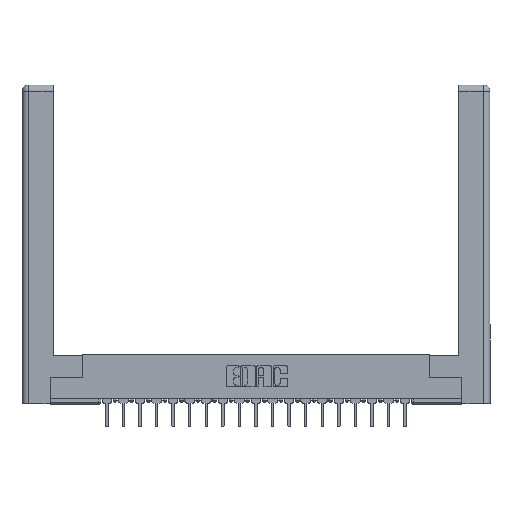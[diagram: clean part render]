
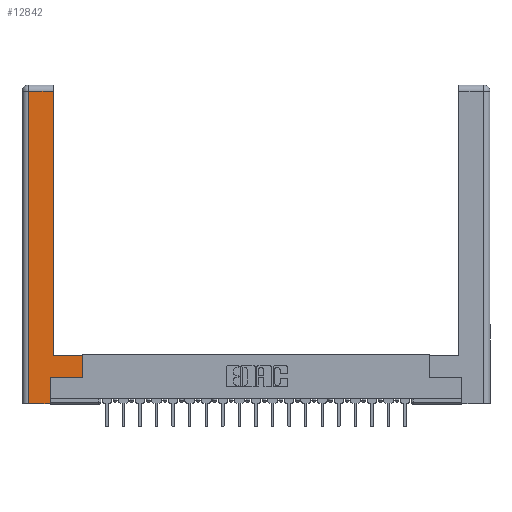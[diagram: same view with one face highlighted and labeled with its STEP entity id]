
A CAD part, top view. The second image highlights one B-rep face of the part: STEP entity #12842.
In plain terms, the highlighted planar face has unit normal (0, 0, 1).
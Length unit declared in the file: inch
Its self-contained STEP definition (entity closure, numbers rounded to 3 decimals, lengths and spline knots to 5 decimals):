
#192 = DIRECTION ( 'NONE',  ( 0., 1., 0. ) ) ;
#274 = CARTESIAN_POINT ( 'NONE',  ( 0.0615, 2.94, 0. ) ) ;
#944 = EDGE_CURVE ( 'NONE', #20094, #19150, #2194, .T. ) ;
#992 = ORIENTED_EDGE ( 'NONE', *, *, #944, .T. ) ;
#1923 = LINE ( 'NONE', #274, #16390 ) ;
#2165 = VERTEX_POINT ( 'NONE', #3200 ) ;
#2194 = LINE ( 'NONE', #18805, #19757 ) ;
#3169 = DIRECTION ( 'NONE',  ( 0., 1., 0. ) ) ;
#3200 = CARTESIAN_POINT ( 'NONE',  ( 0.295, 0.45, 0. ) ) ;
#3791 = VERTEX_POINT ( 'NONE', #3853 ) ;
#3798 = VECTOR ( 'NONE', #8963, 39.37008 ) ;
#3853 = CARTESIAN_POINT ( 'NONE',  ( 0.565, 0.45, 0. ) ) ;
#4119 = ORIENTED_EDGE ( 'NONE', *, *, #5459, .T. ) ;
#4255 = DIRECTION ( 'NONE',  ( -1., 0., 0. ) ) ;
#4571 = LINE ( 'NONE', #21619, #7076 ) ;
#4575 = AXIS2_PLACEMENT_3D ( 'NONE', #20963, #14047, #4255 ) ;
#5139 = CARTESIAN_POINT ( 'NONE',  ( 0.565, 0.45, 0. ) ) ;
#5329 = DIRECTION ( 'NONE',  ( -1., 0., 0. ) ) ;
#5459 = EDGE_CURVE ( 'NONE', #17922, #3791, #18551, .T. ) ;
#5781 = ORIENTED_EDGE ( 'NONE', *, *, #20452, .T. ) ;
#5786 = CARTESIAN_POINT ( 'NONE',  ( 0.265, 0., 0. ) ) ;
#7076 = VECTOR ( 'NONE', #18305, 39.37008 ) ;
#7236 = DIRECTION ( 'NONE',  ( 0., -1., 0. ) ) ;
#8323 = LINE ( 'NONE', #21647, #14307 ) ;
#8963 = DIRECTION ( 'NONE',  ( 1., 0., 0. ) ) ;
#9076 = PLANE ( 'NONE',  #4575 ) ;
#9353 = ORIENTED_EDGE ( 'NONE', *, *, #12625, .T. ) ;
#10151 = VECTOR ( 'NONE', #3169, 39.37008 ) ;
#10496 = ORIENTED_EDGE ( 'NONE', *, *, #21277, .T. ) ;
#11193 = CARTESIAN_POINT ( 'NONE',  ( 0.565, 0.245, 0. ) ) ;
#11832 = CARTESIAN_POINT ( 'NONE',  ( 0.295, 3., 0. ) ) ;
#12067 = LINE ( 'NONE', #5786, #3798 ) ;
#12101 = VECTOR ( 'NONE', #15718, 39.37008 ) ;
#12369 = EDGE_LOOP ( 'NONE', ( #9353, #5781, #992, #10496, #17065, #19643, #4119, #13380 ) ) ;
#12410 = EDGE_CURVE ( 'NONE', #20444, #17922, #19225, .T. ) ;
#12625 = EDGE_CURVE ( 'NONE', #2165, #19174, #13497, .T. ) ;
#12750 = CARTESIAN_POINT ( 'NONE',  ( 0.265, 0., 0. ) ) ;
#12842 = ADVANCED_FACE ( 'NONE', ( #19311 ), #9076, .F. ) ;
#13183 = CARTESIAN_POINT ( 'NONE',  ( 0.295, 2.94, 0. ) ) ;
#13288 = DIRECTION ( 'NONE',  ( -1., 0., 0. ) ) ;
#13380 = ORIENTED_EDGE ( 'NONE', *, *, #19402, .T. ) ;
#13497 = LINE ( 'NONE', #11832, #15985 ) ;
#14047 = DIRECTION ( 'NONE',  ( 0., 0., -1. ) ) ;
#14307 = VECTOR ( 'NONE', #13288, 39.37008 ) ;
#15547 = EDGE_CURVE ( 'NONE', #20928, #20444, #4571, .T. ) ;
#15718 = DIRECTION ( 'NONE',  ( 1., 0., 0. ) ) ;
#15985 = VECTOR ( 'NONE', #192, 39.37008 ) ;
#16390 = VECTOR ( 'NONE', #5329, 39.37008 ) ;
#16982 = CARTESIAN_POINT ( 'NONE',  ( 0.265, 0.245, 0. ) ) ;
#17065 = ORIENTED_EDGE ( 'NONE', *, *, #15547, .T. ) ;
#17922 = VERTEX_POINT ( 'NONE', #11193 ) ;
#18305 = DIRECTION ( 'NONE',  ( 0., 1., 0. ) ) ;
#18551 = LINE ( 'NONE', #5139, #10151 ) ;
#18805 = CARTESIAN_POINT ( 'NONE',  ( 0.0615, 0., 0. ) ) ;
#19150 = VERTEX_POINT ( 'NONE', #21530 ) ;
#19174 = VERTEX_POINT ( 'NONE', #13183 ) ;
#19225 = LINE ( 'NONE', #20666, #12101 ) ;
#19311 = FACE_OUTER_BOUND ( 'NONE', #12369, .T. ) ;
#19402 = EDGE_CURVE ( 'NONE', #3791, #2165, #8323, .T. ) ;
#19643 = ORIENTED_EDGE ( 'NONE', *, *, #12410, .T. ) ;
#19757 = VECTOR ( 'NONE', #7236, 39.37008 ) ;
#20094 = VERTEX_POINT ( 'NONE', #20844 ) ;
#20444 = VERTEX_POINT ( 'NONE', #16982 ) ;
#20452 = EDGE_CURVE ( 'NONE', #19174, #20094, #1923, .T. ) ;
#20666 = CARTESIAN_POINT ( 'NONE',  ( 0.565, 0.245, 0. ) ) ;
#20844 = CARTESIAN_POINT ( 'NONE',  ( 0.0615, 2.94, 0. ) ) ;
#20928 = VERTEX_POINT ( 'NONE', #12750 ) ;
#20963 = CARTESIAN_POINT ( 'NONE',  ( 0., 0., 0. ) ) ;
#21277 = EDGE_CURVE ( 'NONE', #19150, #20928, #12067, .T. ) ;
#21530 = CARTESIAN_POINT ( 'NONE',  ( 0.0615, 0., 0. ) ) ;
#21619 = CARTESIAN_POINT ( 'NONE',  ( 0.265, 0.245, 0. ) ) ;
#21647 = CARTESIAN_POINT ( 'NONE',  ( 0.295, 0.45, 0. ) ) ;
